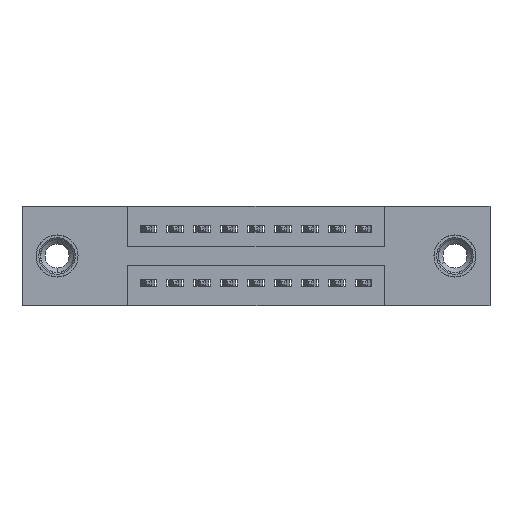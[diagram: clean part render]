
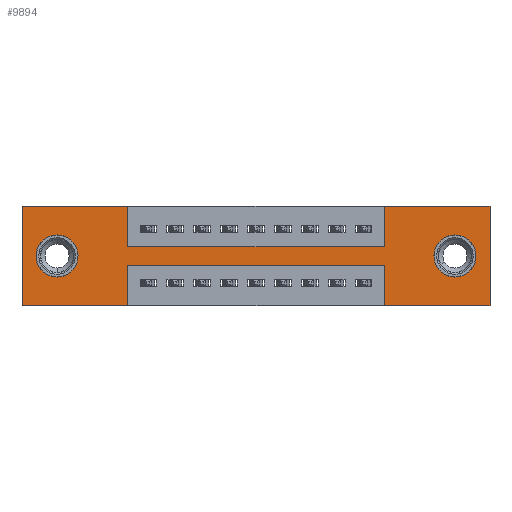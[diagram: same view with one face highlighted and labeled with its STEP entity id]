
A CAD part, front view. The second image highlights one B-rep face of the part: STEP entity #9894.
In plain terms, the highlighted planar face has unit normal (0, -1, 0).
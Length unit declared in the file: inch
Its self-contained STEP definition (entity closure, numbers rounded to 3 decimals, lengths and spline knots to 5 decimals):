
#35 = VERTEX_POINT ( 'NONE', #8309 ) ;
#381 = DIRECTION ( 'NONE',  ( 0., -1., 0. ) ) ;
#539 = EDGE_LOOP ( 'NONE', ( #10068, #7401 ) ) ;
#560 = EDGE_CURVE ( 'NONE', #5003, #35, #2838, .T. ) ;
#948 = DIRECTION ( 'NONE',  ( -1., 0., 0. ) ) ;
#1009 = CARTESIAN_POINT ( 'NONE',  ( 1.605, 0., -0.185 ) ) ;
#1109 = LINE ( 'NONE', #7895, #7122 ) ;
#1118 = VECTOR ( 'NONE', #948, 39.37008 ) ;
#1132 = EDGE_CURVE ( 'NONE', #9107, #8683, #1109, .T. ) ;
#1235 = FACE_BOUND ( 'NONE', #539, .T. ) ;
#1238 = VERTEX_POINT ( 'NONE', #8084 ) ;
#1353 = VERTEX_POINT ( 'NONE', #6988 ) ;
#1513 = DIRECTION ( 'NONE',  ( 0., 1., 0. ) ) ;
#1629 = VECTOR ( 'NONE', #8368, 39.37008 ) ;
#1670 = LINE ( 'NONE', #11075, #3335 ) ;
#1929 = VERTEX_POINT ( 'NONE', #6514 ) ;
#1972 = CARTESIAN_POINT ( 'NONE',  ( 0., 0., 0. ) ) ;
#2346 = ORIENTED_EDGE ( 'NONE', *, *, #10016, .T. ) ;
#2391 = CIRCLE ( 'NONE', #7139, 0.078 ) ;
#2422 = ORIENTED_EDGE ( 'NONE', *, *, #12463, .F. ) ;
#2436 = EDGE_LOOP ( 'NONE', ( #10037, #2868, #6064, #11770, #3748, #4801, #9481, #2422, #12585, #5292, #11421, #2876 ) ) ;
#2571 = DIRECTION ( 'NONE',  ( 0., 0., -1. ) ) ;
#2615 = CARTESIAN_POINT ( 'NONE',  ( 1.735, 0., 0. ) ) ;
#2814 = DIRECTION ( 'NONE',  ( 0., 0., 1. ) ) ;
#2838 = CIRCLE ( 'NONE', #8667, 0.078 ) ;
#2868 = ORIENTED_EDGE ( 'NONE', *, *, #5746, .F. ) ;
#2876 = ORIENTED_EDGE ( 'NONE', *, *, #7864, .F. ) ;
#2894 = CARTESIAN_POINT ( 'NONE',  ( 0., 0., -0.37 ) ) ;
#2905 = LINE ( 'NONE', #6581, #3674 ) ;
#3065 = CIRCLE ( 'NONE', #8338, 0.078 ) ;
#3089 = CARTESIAN_POINT ( 'NONE',  ( 0.3925, 0., -0.22 ) ) ;
#3118 = AXIS2_PLACEMENT_3D ( 'NONE', #4398, #381, #8187 ) ;
#3121 = CARTESIAN_POINT ( 'NONE',  ( 1.735, 0., 0. ) ) ;
#3186 = EDGE_CURVE ( 'NONE', #5606, #9875, #2905, .T. ) ;
#3227 = CARTESIAN_POINT ( 'NONE',  ( 1.3425, 0., -0.37 ) ) ;
#3335 = VECTOR ( 'NONE', #11251, 39.37008 ) ;
#3439 = LINE ( 'NONE', #6778, #11733 ) ;
#3543 = VERTEX_POINT ( 'NONE', #8010 ) ;
#3605 = CIRCLE ( 'NONE', #4066, 0.078 ) ;
#3671 = CARTESIAN_POINT ( 'NONE',  ( 0.3925, 0., 0. ) ) ;
#3674 = VECTOR ( 'NONE', #6540, 39.37008 ) ;
#3728 = LINE ( 'NONE', #2894, #1118 ) ;
#3748 = ORIENTED_EDGE ( 'NONE', *, *, #8470, .F. ) ;
#3757 = CARTESIAN_POINT ( 'NONE',  ( 1.3425, 0., 0. ) ) ;
#4044 = DIRECTION ( 'NONE',  ( 1., 0., 0. ) ) ;
#4066 = AXIS2_PLACEMENT_3D ( 'NONE', #6267, #8093, #12037 ) ;
#4182 = CARTESIAN_POINT ( 'NONE',  ( 0.3925, 0., -0.15 ) ) ;
#4371 = CARTESIAN_POINT ( 'NONE',  ( 1.605, 0., -0.185 ) ) ;
#4398 = CARTESIAN_POINT ( 'NONE',  ( 0., 0., -0.37 ) ) ;
#4688 = LINE ( 'NONE', #3227, #1629 ) ;
#4787 = EDGE_CURVE ( 'NONE', #3543, #10650, #4688, .T. ) ;
#4801 = ORIENTED_EDGE ( 'NONE', *, *, #3186, .F. ) ;
#5003 = VERTEX_POINT ( 'NONE', #5395 ) ;
#5292 = ORIENTED_EDGE ( 'NONE', *, *, #7906, .F. ) ;
#5395 = CARTESIAN_POINT ( 'NONE',  ( 1.605, 0., -0.107 ) ) ;
#5606 = VERTEX_POINT ( 'NONE', #3757 ) ;
#5746 = EDGE_CURVE ( 'NONE', #10650, #6997, #11760, .T. ) ;
#5784 = VECTOR ( 'NONE', #2571, 39.37008 ) ;
#5828 = DIRECTION ( 'NONE',  ( 1., 0., 0. ) ) ;
#6014 = CARTESIAN_POINT ( 'NONE',  ( 0.13, 0., -0.263 ) ) ;
#6064 = ORIENTED_EDGE ( 'NONE', *, *, #4787, .F. ) ;
#6267 = CARTESIAN_POINT ( 'NONE',  ( 0.13, 0., -0.185 ) ) ;
#6514 = CARTESIAN_POINT ( 'NONE',  ( 0.3925, 0., 0. ) ) ;
#6540 = DIRECTION ( 'NONE',  ( 1., 0., 0. ) ) ;
#6581 = CARTESIAN_POINT ( 'NONE',  ( 0., 0., 0. ) ) ;
#6778 = CARTESIAN_POINT ( 'NONE',  ( 0., 0., -0.37 ) ) ;
#6823 = DIRECTION ( 'NONE',  ( 0., 0., -1. ) ) ;
#6846 = EDGE_CURVE ( 'NONE', #8318, #10325, #3605, .T. ) ;
#6914 = EDGE_LOOP ( 'NONE', ( #7982, #2346 ) ) ;
#6988 = CARTESIAN_POINT ( 'NONE',  ( 0.3925, 0., -0.37 ) ) ;
#6997 = VERTEX_POINT ( 'NONE', #11270 ) ;
#7122 = VECTOR ( 'NONE', #2814, 39.37008 ) ;
#7139 = AXIS2_PLACEMENT_3D ( 'NONE', #4371, #1513, #7429 ) ;
#7401 = ORIENTED_EDGE ( 'NONE', *, *, #7611, .T. ) ;
#7429 = DIRECTION ( 'NONE',  ( 0., 0., -1. ) ) ;
#7611 = EDGE_CURVE ( 'NONE', #35, #5003, #2391, .T. ) ;
#7766 = LINE ( 'NONE', #4182, #10538 ) ;
#7864 = EDGE_CURVE ( 'NONE', #1353, #9107, #3439, .T. ) ;
#7895 = CARTESIAN_POINT ( 'NONE',  ( 0., 0., 0. ) ) ;
#7906 = EDGE_CURVE ( 'NONE', #8683, #1929, #8787, .T. ) ;
#7982 = ORIENTED_EDGE ( 'NONE', *, *, #6846, .T. ) ;
#8010 = CARTESIAN_POINT ( 'NONE',  ( 1.3425, 0., -0.37 ) ) ;
#8025 = PLANE ( 'NONE',  #3118 ) ;
#8084 = CARTESIAN_POINT ( 'NONE',  ( 0.3925, 0., -0.15 ) ) ;
#8093 = DIRECTION ( 'NONE',  ( 0., 1., 0. ) ) ;
#8158 = VERTEX_POINT ( 'NONE', #8460 ) ;
#8187 = DIRECTION ( 'NONE',  ( 0., 0., -1. ) ) ;
#8263 = DIRECTION ( 'NONE',  ( 0., 0., 1. ) ) ;
#8309 = CARTESIAN_POINT ( 'NONE',  ( 1.605, 0., -0.263 ) ) ;
#8318 = VERTEX_POINT ( 'NONE', #9270 ) ;
#8338 = AXIS2_PLACEMENT_3D ( 'NONE', #12134, #9099, #8263 ) ;
#8368 = DIRECTION ( 'NONE',  ( 0., 0., 1. ) ) ;
#8460 = CARTESIAN_POINT ( 'NONE',  ( 1.735, 0., -0.37 ) ) ;
#8470 = EDGE_CURVE ( 'NONE', #9875, #8158, #8778, .T. ) ;
#8573 = DIRECTION ( 'NONE',  ( 0., 0., -1. ) ) ;
#8651 = LINE ( 'NONE', #3671, #5784 ) ;
#8667 = AXIS2_PLACEMENT_3D ( 'NONE', #1009, #10825, #6823 ) ;
#8683 = VERTEX_POINT ( 'NONE', #8730 ) ;
#8721 = FACE_OUTER_BOUND ( 'NONE', #2436, .T. ) ;
#8730 = CARTESIAN_POINT ( 'NONE',  ( 0., 0., 0. ) ) ;
#8734 = EDGE_CURVE ( 'NONE', #8158, #3543, #3728, .T. ) ;
#8778 = LINE ( 'NONE', #2615, #9566 ) ;
#8787 = LINE ( 'NONE', #1972, #10798 ) ;
#8819 = DIRECTION ( 'NONE',  ( -1., 0., 0. ) ) ;
#9013 = CARTESIAN_POINT ( 'NONE',  ( 0., 0., -0.37 ) ) ;
#9092 = DIRECTION ( 'NONE',  ( 0., 0., -1. ) ) ;
#9099 = DIRECTION ( 'NONE',  ( 0., 1., 0. ) ) ;
#9107 = VERTEX_POINT ( 'NONE', #9013 ) ;
#9270 = CARTESIAN_POINT ( 'NONE',  ( 0.13, 0., -0.107 ) ) ;
#9450 = CARTESIAN_POINT ( 'NONE',  ( 1.3425, 0., -0.22 ) ) ;
#9481 = ORIENTED_EDGE ( 'NONE', *, *, #11715, .F. ) ;
#9566 = VECTOR ( 'NONE', #8573, 39.37008 ) ;
#9633 = CARTESIAN_POINT ( 'NONE',  ( 1.3425, 0., -0.15 ) ) ;
#9757 = DIRECTION ( 'NONE',  ( -1., 0., 0. ) ) ;
#9875 = VERTEX_POINT ( 'NONE', #3121 ) ;
#9894 = ADVANCED_FACE ( 'NONE', ( #1235, #12621, #8721 ), #8025, .T. ) ;
#10016 = EDGE_CURVE ( 'NONE', #10325, #8318, #3065, .T. ) ;
#10037 = ORIENTED_EDGE ( 'NONE', *, *, #12386, .F. ) ;
#10068 = ORIENTED_EDGE ( 'NONE', *, *, #560, .T. ) ;
#10218 = VECTOR ( 'NONE', #9092, 39.37008 ) ;
#10222 = VERTEX_POINT ( 'NONE', #9633 ) ;
#10325 = VERTEX_POINT ( 'NONE', #6014 ) ;
#10538 = VECTOR ( 'NONE', #4044, 39.37008 ) ;
#10543 = LINE ( 'NONE', #10924, #10218 ) ;
#10650 = VERTEX_POINT ( 'NONE', #9450 ) ;
#10695 = VECTOR ( 'NONE', #8819, 39.37008 ) ;
#10798 = VECTOR ( 'NONE', #5828, 39.37008 ) ;
#10825 = DIRECTION ( 'NONE',  ( 0., 1., 0. ) ) ;
#10924 = CARTESIAN_POINT ( 'NONE',  ( 0.3925, 0., -0.37 ) ) ;
#11075 = CARTESIAN_POINT ( 'NONE',  ( 1.3425, 0., 0. ) ) ;
#11251 = DIRECTION ( 'NONE',  ( 0., 0., 1. ) ) ;
#11270 = CARTESIAN_POINT ( 'NONE',  ( 0.3925, 0., -0.22 ) ) ;
#11421 = ORIENTED_EDGE ( 'NONE', *, *, #1132, .F. ) ;
#11715 = EDGE_CURVE ( 'NONE', #10222, #5606, #1670, .T. ) ;
#11733 = VECTOR ( 'NONE', #9757, 39.37008 ) ;
#11760 = LINE ( 'NONE', #3089, #10695 ) ;
#11770 = ORIENTED_EDGE ( 'NONE', *, *, #8734, .F. ) ;
#12037 = DIRECTION ( 'NONE',  ( 0., 0., 1. ) ) ;
#12134 = CARTESIAN_POINT ( 'NONE',  ( 0.13, 0., -0.185 ) ) ;
#12386 = EDGE_CURVE ( 'NONE', #6997, #1353, #10543, .T. ) ;
#12463 = EDGE_CURVE ( 'NONE', #1238, #10222, #7766, .T. ) ;
#12585 = ORIENTED_EDGE ( 'NONE', *, *, #12608, .F. ) ;
#12608 = EDGE_CURVE ( 'NONE', #1929, #1238, #8651, .T. ) ;
#12621 = FACE_BOUND ( 'NONE', #6914, .T. ) ;
